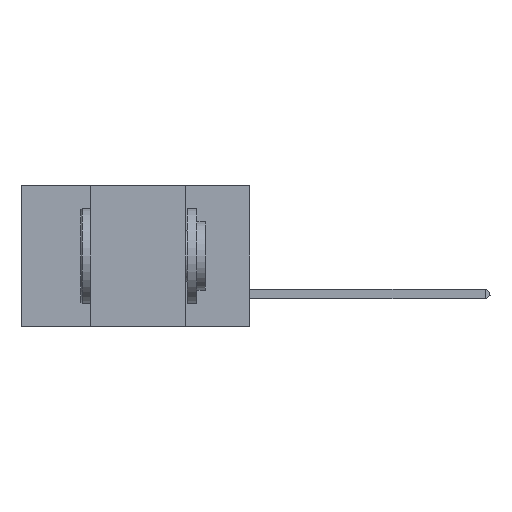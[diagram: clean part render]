
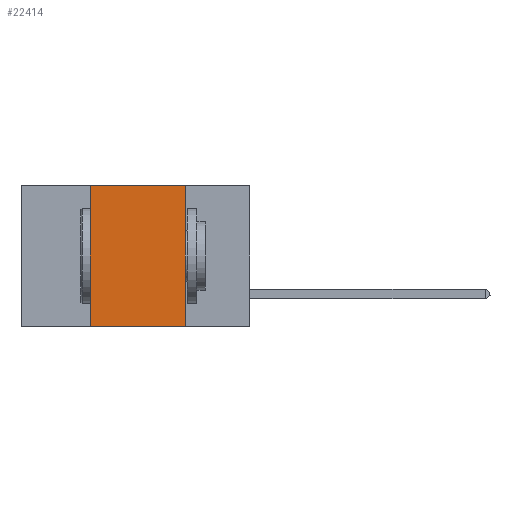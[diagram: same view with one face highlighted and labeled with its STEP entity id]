
A CAD part, left-side view. The second image highlights one B-rep face of the part: STEP entity #22414.
In plain terms, the highlighted planar face has unit normal (-1, 0, 0).
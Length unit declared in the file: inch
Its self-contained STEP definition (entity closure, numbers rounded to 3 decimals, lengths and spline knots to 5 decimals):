
#929 = CARTESIAN_POINT ( 'NONE',  ( 0., 0.17, 0. ) ) ;
#1323 = FACE_OUTER_BOUND ( 'NONE', #9431, .T. ) ;
#2439 = CARTESIAN_POINT ( 'NONE',  ( 0., 0.6, -0.37 ) ) ;
#4457 = PLANE ( 'NONE',  #23709 ) ;
#7371 = ORIENTED_EDGE ( 'NONE', *, *, #18883, .T. ) ;
#7602 = CARTESIAN_POINT ( 'NONE',  ( 0., 0.42, -0.37 ) ) ;
#7939 = VERTEX_POINT ( 'NONE', #14772 ) ;
#8463 = DIRECTION ( 'NONE',  ( 0., 0., -1. ) ) ;
#8864 = EDGE_CURVE ( 'NONE', #14868, #23049, #22614, .T. ) ;
#8952 = CARTESIAN_POINT ( 'NONE',  ( 0., 0.42, 0. ) ) ;
#9118 = DIRECTION ( 'NONE',  ( 0., 0., 1. ) ) ;
#9431 = EDGE_LOOP ( 'NONE', ( #25006, #21493, #26002, #7371 ) ) ;
#9701 = DIRECTION ( 'NONE',  ( 0., -1., 0. ) ) ;
#10454 = DIRECTION ( 'NONE',  ( 1., 0., 0. ) ) ;
#12527 = LINE ( 'NONE', #26358, #26455 ) ;
#12580 = DIRECTION ( 'NONE',  ( 0., -1., 0. ) ) ;
#14772 = CARTESIAN_POINT ( 'NONE',  ( 0., 0.17, 0. ) ) ;
#14868 = VERTEX_POINT ( 'NONE', #7602 ) ;
#15063 = VECTOR ( 'NONE', #23705, 39.37008 ) ;
#15870 = CARTESIAN_POINT ( 'NONE',  ( 0., 0.42, 0. ) ) ;
#17094 = LINE ( 'NONE', #2439, #21022 ) ;
#18694 = CARTESIAN_POINT ( 'NONE',  ( 0., 0.6, 0. ) ) ;
#18883 = EDGE_CURVE ( 'NONE', #14868, #25543, #17094, .T. ) ;
#19546 = EDGE_CURVE ( 'NONE', #23049, #7939, #12527, .T. ) ;
#20615 = LINE ( 'NONE', #929, #15063 ) ;
#20685 = EDGE_CURVE ( 'NONE', #7939, #25543, #20615, .T. ) ;
#21022 = VECTOR ( 'NONE', #12580, 39.37008 ) ;
#21493 = ORIENTED_EDGE ( 'NONE', *, *, #19546, .F. ) ;
#22414 = ADVANCED_FACE ( 'NONE', ( #1323 ), #4457, .F. ) ;
#22614 = LINE ( 'NONE', #8952, #26795 ) ;
#23049 = VERTEX_POINT ( 'NONE', #15870 ) ;
#23705 = DIRECTION ( 'NONE',  ( 0., 0., -1. ) ) ;
#23709 = AXIS2_PLACEMENT_3D ( 'NONE', #18694, #10454, #8463 ) ;
#25006 = ORIENTED_EDGE ( 'NONE', *, *, #20685, .F. ) ;
#25459 = CARTESIAN_POINT ( 'NONE',  ( 0., 0.17, -0.37 ) ) ;
#25543 = VERTEX_POINT ( 'NONE', #25459 ) ;
#26002 = ORIENTED_EDGE ( 'NONE', *, *, #8864, .F. ) ;
#26358 = CARTESIAN_POINT ( 'NONE',  ( 0., 0.6, 0. ) ) ;
#26455 = VECTOR ( 'NONE', #9701, 39.37008 ) ;
#26795 = VECTOR ( 'NONE', #9118, 39.37008 ) ;
